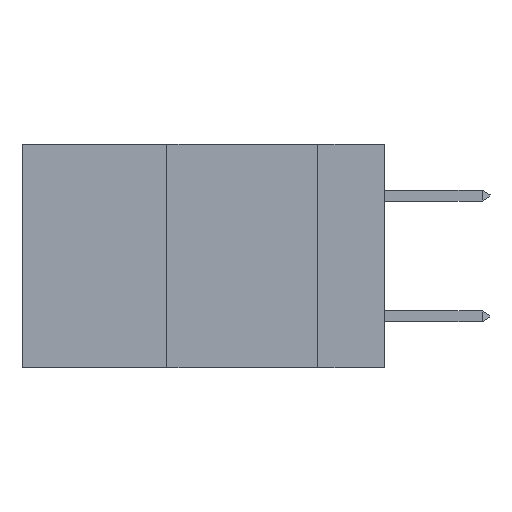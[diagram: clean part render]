
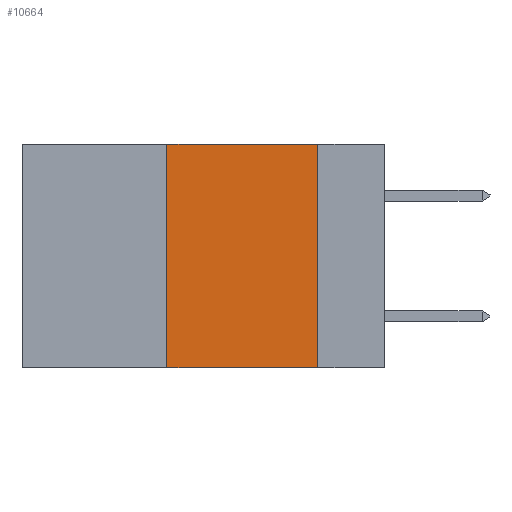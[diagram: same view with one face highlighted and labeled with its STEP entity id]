
A CAD part, left-side view. The second image highlights one B-rep face of the part: STEP entity #10664.
In plain terms, the highlighted planar face has unit normal (-1, 0, 0).
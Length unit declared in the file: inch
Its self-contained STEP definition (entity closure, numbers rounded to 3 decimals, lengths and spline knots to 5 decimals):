
#248 = DIRECTION ( 'NONE',  ( 0., -1., 0. ) ) ;
#1045 = CARTESIAN_POINT ( 'NONE',  ( 0., 0.36, 0. ) ) ;
#2099 = VERTEX_POINT ( 'NONE', #3793 ) ;
#3793 = CARTESIAN_POINT ( 'NONE',  ( 0., 0.36, -0.37 ) ) ;
#4541 = EDGE_CURVE ( 'NONE', #11845, #10585, #23367, .T. ) ;
#4882 = DIRECTION ( 'NONE',  ( 0., 0., 1. ) ) ;
#5179 = PLANE ( 'NONE',  #9401 ) ;
#5256 = VERTEX_POINT ( 'NONE', #25357 ) ;
#5930 = DIRECTION ( 'NONE',  ( 0., 0., -1. ) ) ;
#6790 = VECTOR ( 'NONE', #5930, 39.37008 ) ;
#6987 = CARTESIAN_POINT ( 'NONE',  ( 0., 0.36, 0. ) ) ;
#9075 = ORIENTED_EDGE ( 'NONE', *, *, #11020, .F. ) ;
#9087 = LINE ( 'NONE', #18500, #6790 ) ;
#9211 = LINE ( 'NONE', #6987, #23992 ) ;
#9401 = AXIS2_PLACEMENT_3D ( 'NONE', #26741, #11944, #18560 ) ;
#9643 = CARTESIAN_POINT ( 'NONE',  ( 0., 0.6, 0. ) ) ;
#10585 = VERTEX_POINT ( 'NONE', #13788 ) ;
#10664 = ADVANCED_FACE ( 'NONE', ( #22053 ), #5179, .F. ) ;
#11020 = EDGE_CURVE ( 'NONE', #2099, #11845, #9211, .T. ) ;
#11752 = DIRECTION ( 'NONE',  ( 0., -1., 0. ) ) ;
#11845 = VERTEX_POINT ( 'NONE', #1045 ) ;
#11944 = DIRECTION ( 'NONE',  ( 1., 0., 0. ) ) ;
#12719 = EDGE_CURVE ( 'NONE', #10585, #5256, #9087, .T. ) ;
#13788 = CARTESIAN_POINT ( 'NONE',  ( 0., 0.11, 0. ) ) ;
#13899 = LINE ( 'NONE', #23175, #20506 ) ;
#15278 = EDGE_CURVE ( 'NONE', #2099, #5256, #13899, .T. ) ;
#15756 = ORIENTED_EDGE ( 'NONE', *, *, #4541, .F. ) ;
#18101 = VECTOR ( 'NONE', #11752, 39.37008 ) ;
#18500 = CARTESIAN_POINT ( 'NONE',  ( 0., 0.11, 0. ) ) ;
#18560 = DIRECTION ( 'NONE',  ( 0., 0., -1. ) ) ;
#20506 = VECTOR ( 'NONE', #248, 39.37008 ) ;
#22053 = FACE_OUTER_BOUND ( 'NONE', #26076, .T. ) ;
#23175 = CARTESIAN_POINT ( 'NONE',  ( 0., 0.6, -0.37 ) ) ;
#23367 = LINE ( 'NONE', #9643, #18101 ) ;
#23992 = VECTOR ( 'NONE', #4882, 39.37008 ) ;
#25357 = CARTESIAN_POINT ( 'NONE',  ( 0., 0.11, -0.37 ) ) ;
#26076 = EDGE_LOOP ( 'NONE', ( #26097, #15756, #9075, #26100 ) ) ;
#26097 = ORIENTED_EDGE ( 'NONE', *, *, #12719, .F. ) ;
#26100 = ORIENTED_EDGE ( 'NONE', *, *, #15278, .T. ) ;
#26741 = CARTESIAN_POINT ( 'NONE',  ( 0., 0.6, 0. ) ) ;
